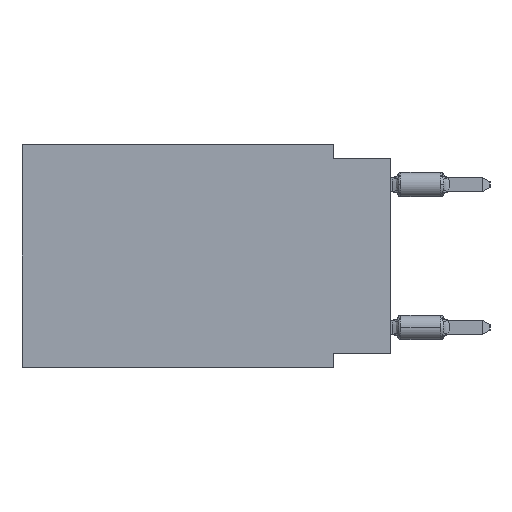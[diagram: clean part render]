
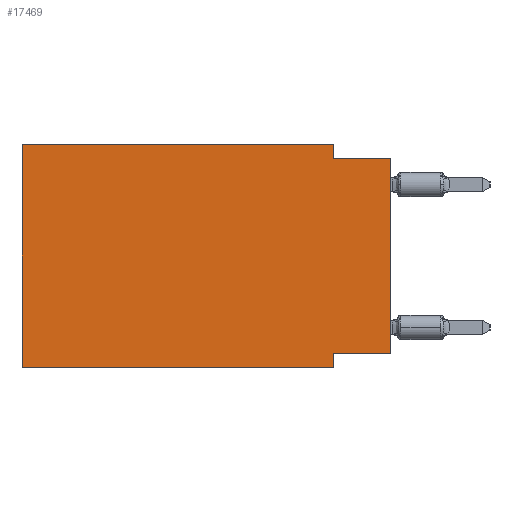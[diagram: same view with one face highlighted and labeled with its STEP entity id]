
A CAD part, left-side view. The second image highlights one B-rep face of the part: STEP entity #17469.
In plain terms, the highlighted planar face has unit normal (-1, 0, 0).
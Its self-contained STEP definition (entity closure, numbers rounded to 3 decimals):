
#254 = VECTOR ( 'NONE', #1686, 1000. ) ;
#727 = VECTOR ( 'NONE', #24602, 1000. ) ;
#1350 = CARTESIAN_POINT ( 'NONE',  ( 0., 0., 0. ) ) ;
#1686 = DIRECTION ( 'NONE',  ( 0., -1., 0. ) ) ;
#1815 = ORIENTED_EDGE ( 'NONE', *, *, #23955, .F. ) ;
#2167 = CARTESIAN_POINT ( 'NONE',  ( 0., 2.54, -9.906 ) ) ;
#2892 = ORIENTED_EDGE ( 'NONE', *, *, #19161, .F. ) ;
#3468 = VECTOR ( 'NONE', #4262, 1000. ) ;
#4042 = LINE ( 'NONE', #1350, #7593 ) ;
#4262 = DIRECTION ( 'NONE',  ( 0., 0., 1. ) ) ;
#4826 = EDGE_CURVE ( 'NONE', #24594, #15181, #10089, .T. ) ;
#5583 = CARTESIAN_POINT ( 'NONE',  ( 0., 2.54, -9.906 ) ) ;
#6065 = DIRECTION ( 'NONE',  ( 0., 0., -1. ) ) ;
#6205 = LINE ( 'NONE', #5583, #6971 ) ;
#6227 = DIRECTION ( 'NONE',  ( 0., -1., 0. ) ) ;
#6310 = CARTESIAN_POINT ( 'NONE',  ( 0., 0., -0.635 ) ) ;
#6384 = ORIENTED_EDGE ( 'NONE', *, *, #7284, .F. ) ;
#6640 = CARTESIAN_POINT ( 'NONE',  ( 0., 16.383, 0. ) ) ;
#6971 = VECTOR ( 'NONE', #15492, 1000. ) ;
#7284 = EDGE_CURVE ( 'NONE', #12019, #27440, #27827, .T. ) ;
#7593 = VECTOR ( 'NONE', #27384, 1000. ) ;
#8297 = ORIENTED_EDGE ( 'NONE', *, *, #24502, .T. ) ;
#9259 = CARTESIAN_POINT ( 'NONE',  ( 0., 16.383, 0. ) ) ;
#9775 = VERTEX_POINT ( 'NONE', #22465 ) ;
#9826 = LINE ( 'NONE', #9982, #14191 ) ;
#9982 = CARTESIAN_POINT ( 'NONE',  ( 0., 0., -9.271 ) ) ;
#10089 = LINE ( 'NONE', #22052, #10536 ) ;
#10536 = VECTOR ( 'NONE', #11974, 1000. ) ;
#11220 = DIRECTION ( 'NONE',  ( 0., 1., 0. ) ) ;
#11974 = DIRECTION ( 'NONE',  ( 0., -1., 0. ) ) ;
#12019 = VERTEX_POINT ( 'NONE', #22197 ) ;
#13039 = EDGE_CURVE ( 'NONE', #28254, #15322, #6205, .T. ) ;
#13561 = LINE ( 'NONE', #6640, #3468 ) ;
#13644 = EDGE_CURVE ( 'NONE', #9775, #24594, #13561, .T. ) ;
#13928 = CARTESIAN_POINT ( 'NONE',  ( 0., 0., -0.635 ) ) ;
#14191 = VECTOR ( 'NONE', #11220, 1000. ) ;
#15181 = VERTEX_POINT ( 'NONE', #18260 ) ;
#15322 = VERTEX_POINT ( 'NONE', #2167 ) ;
#15492 = DIRECTION ( 'NONE',  ( 0., 0., -1. ) ) ;
#15783 = EDGE_LOOP ( 'NONE', ( #15999, #6384, #1815, #23114, #19098, #8297, #24310, #2892 ) ) ;
#15795 = VERTEX_POINT ( 'NONE', #29987 ) ;
#15892 = EDGE_CURVE ( 'NONE', #15795, #27440, #4042, .T. ) ;
#15999 = ORIENTED_EDGE ( 'NONE', *, *, #15892, .T. ) ;
#16638 = AXIS2_PLACEMENT_3D ( 'NONE', #18027, #25592, #6065 ) ;
#17469 = ADVANCED_FACE ( 'NONE', ( #27505 ), #20252, .F. ) ;
#18027 = CARTESIAN_POINT ( 'NONE',  ( 0., 16.383, 0. ) ) ;
#18260 = CARTESIAN_POINT ( 'NONE',  ( 0., 2.54, 0. ) ) ;
#19098 = ORIENTED_EDGE ( 'NONE', *, *, #13644, .F. ) ;
#19161 = EDGE_CURVE ( 'NONE', #15795, #28254, #9826, .T. ) ;
#20252 = PLANE ( 'NONE',  #16638 ) ;
#22052 = CARTESIAN_POINT ( 'NONE',  ( 0., 16.383, 0. ) ) ;
#22197 = CARTESIAN_POINT ( 'NONE',  ( 0., 2.54, -0.635 ) ) ;
#22234 = CARTESIAN_POINT ( 'NONE',  ( 0., 2.54, 0. ) ) ;
#22465 = CARTESIAN_POINT ( 'NONE',  ( 0., 16.383, -9.906 ) ) ;
#23114 = ORIENTED_EDGE ( 'NONE', *, *, #4826, .F. ) ;
#23955 = EDGE_CURVE ( 'NONE', #15181, #12019, #28883, .T. ) ;
#24310 = ORIENTED_EDGE ( 'NONE', *, *, #13039, .F. ) ;
#24502 = EDGE_CURVE ( 'NONE', #9775, #15322, #30873, .T. ) ;
#24594 = VERTEX_POINT ( 'NONE', #9259 ) ;
#24602 = DIRECTION ( 'NONE',  ( 0., 0., -1. ) ) ;
#24683 = CARTESIAN_POINT ( 'NONE',  ( 0., 2.54, -9.271 ) ) ;
#25592 = DIRECTION ( 'NONE',  ( 1., 0., 0. ) ) ;
#27384 = DIRECTION ( 'NONE',  ( 0., 0., 1. ) ) ;
#27440 = VERTEX_POINT ( 'NONE', #6310 ) ;
#27505 = FACE_OUTER_BOUND ( 'NONE', #15783, .T. ) ;
#27827 = LINE ( 'NONE', #13928, #30193 ) ;
#28254 = VERTEX_POINT ( 'NONE', #24683 ) ;
#28883 = LINE ( 'NONE', #22234, #727 ) ;
#29987 = CARTESIAN_POINT ( 'NONE',  ( 0., 0., -9.271 ) ) ;
#30193 = VECTOR ( 'NONE', #6227, 1000. ) ;
#30254 = CARTESIAN_POINT ( 'NONE',  ( 0., 16.383, -9.906 ) ) ;
#30873 = LINE ( 'NONE', #30254, #254 ) ;
